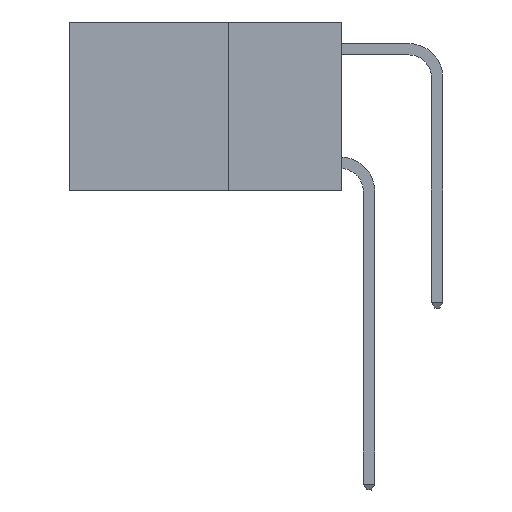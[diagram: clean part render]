
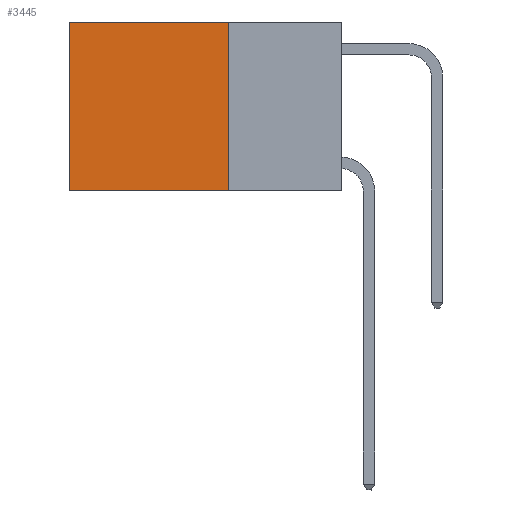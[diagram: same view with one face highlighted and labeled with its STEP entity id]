
A CAD part, left-side view. The second image highlights one B-rep face of the part: STEP entity #3445.
In plain terms, the highlighted planar face has unit normal (-1, 0, 0).
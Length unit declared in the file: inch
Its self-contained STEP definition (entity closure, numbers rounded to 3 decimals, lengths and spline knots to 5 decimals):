
#18 = LINE ( 'NONE', #3216, #1463 ) ;
#784 = EDGE_CURVE ( 'NONE', #1762, #10562, #8418, .T. ) ;
#1289 = ORIENTED_EDGE ( 'NONE', *, *, #784, .T. ) ;
#1463 = VECTOR ( 'NONE', #6170, 39.37008 ) ;
#1626 = PLANE ( 'NONE',  #5054 ) ;
#1762 = VERTEX_POINT ( 'NONE', #8023 ) ;
#2241 = DIRECTION ( 'NONE',  ( 0., 0., -1. ) ) ;
#2323 = EDGE_CURVE ( 'NONE', #1762, #4255, #18, .T. ) ;
#2531 = LINE ( 'NONE', #3089, #5169 ) ;
#2576 = EDGE_CURVE ( 'NONE', #10562, #2847, #2531, .T. ) ;
#2847 = VERTEX_POINT ( 'NONE', #6415 ) ;
#3087 = EDGE_LOOP ( 'NONE', ( #4601, #5128, #5397, #1289 ) ) ;
#3089 = CARTESIAN_POINT ( 'NONE',  ( 0.2625, 0.6, 0. ) ) ;
#3216 = CARTESIAN_POINT ( 'NONE',  ( 0.2625, 0.25, 0. ) ) ;
#3445 = ADVANCED_FACE ( 'NONE', ( #5537 ), #1626, .F. ) ;
#4062 = EDGE_CURVE ( 'NONE', #4255, #2847, #6935, .T. ) ;
#4255 = VERTEX_POINT ( 'NONE', #7543 ) ;
#4368 = DIRECTION ( 'NONE',  ( 0., 0., -1. ) ) ;
#4601 = ORIENTED_EDGE ( 'NONE', *, *, #2576, .T. ) ;
#5054 = AXIS2_PLACEMENT_3D ( 'NONE', #6851, #9998, #4368 ) ;
#5128 = ORIENTED_EDGE ( 'NONE', *, *, #4062, .F. ) ;
#5169 = VECTOR ( 'NONE', #2241, 39.37008 ) ;
#5397 = ORIENTED_EDGE ( 'NONE', *, *, #2323, .F. ) ;
#5537 = FACE_OUTER_BOUND ( 'NONE', #3087, .T. ) ;
#6170 = DIRECTION ( 'NONE',  ( 0., 0., -1. ) ) ;
#6240 = VECTOR ( 'NONE', #9787, 39.37008 ) ;
#6415 = CARTESIAN_POINT ( 'NONE',  ( 0.2625, 0.6, -0.37 ) ) ;
#6851 = CARTESIAN_POINT ( 'NONE',  ( 0.2625, 0.25, 0. ) ) ;
#6935 = LINE ( 'NONE', #10304, #10696 ) ;
#7543 = CARTESIAN_POINT ( 'NONE',  ( 0.2625, 0.25, -0.37 ) ) ;
#8023 = CARTESIAN_POINT ( 'NONE',  ( 0.2625, 0.25, 0. ) ) ;
#8418 = LINE ( 'NONE', #9571, #6240 ) ;
#8453 = CARTESIAN_POINT ( 'NONE',  ( 0.2625, 0.6, 0. ) ) ;
#9571 = CARTESIAN_POINT ( 'NONE',  ( 0.2625, 0.25, 0. ) ) ;
#9787 = DIRECTION ( 'NONE',  ( 0., 1., 0. ) ) ;
#9998 = DIRECTION ( 'NONE',  ( 1., 0., 0. ) ) ;
#10304 = CARTESIAN_POINT ( 'NONE',  ( 0.2625, 0.25, -0.37 ) ) ;
#10562 = VERTEX_POINT ( 'NONE', #8453 ) ;
#10696 = VECTOR ( 'NONE', #11073, 39.37008 ) ;
#11073 = DIRECTION ( 'NONE',  ( 0., 1., 0. ) ) ;
